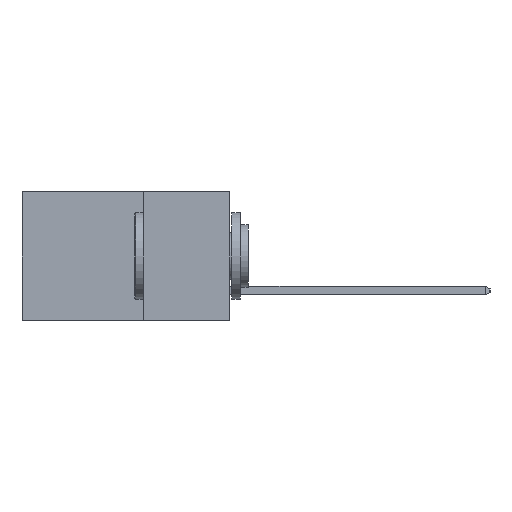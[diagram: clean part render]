
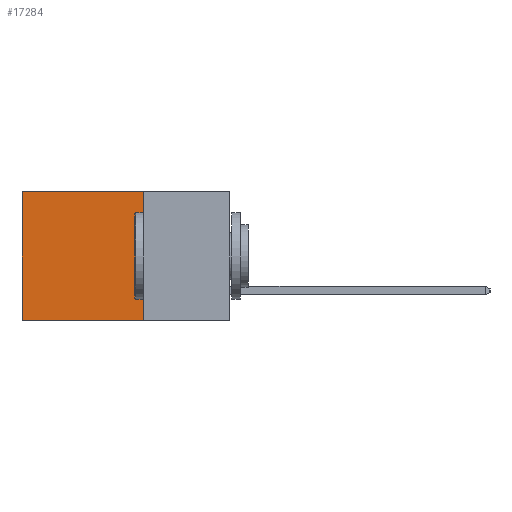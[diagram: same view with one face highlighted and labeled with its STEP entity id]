
A CAD part, left-side view. The second image highlights one B-rep face of the part: STEP entity #17284.
In plain terms, the highlighted planar face has unit normal (-1, 0, 0).
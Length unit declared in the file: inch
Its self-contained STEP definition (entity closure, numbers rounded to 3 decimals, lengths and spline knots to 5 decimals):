
#304 = VERTEX_POINT ( 'NONE', #15848 ) ;
#619 = EDGE_CURVE ( 'NONE', #304, #3793, #16123, .T. ) ;
#997 = FACE_OUTER_BOUND ( 'NONE', #23389, .T. ) ;
#1008 = CARTESIAN_POINT ( 'NONE',  ( 0.2615, 0.6, -0.37 ) ) ;
#1501 = EDGE_CURVE ( 'NONE', #9234, #13480, #11164, .T. ) ;
#1624 = ORIENTED_EDGE ( 'NONE', *, *, #1501, .T. ) ;
#1763 = ORIENTED_EDGE ( 'NONE', *, *, #7703, .T. ) ;
#3793 = VERTEX_POINT ( 'NONE', #11494 ) ;
#4289 = LINE ( 'NONE', #14036, #9132 ) ;
#4417 = VECTOR ( 'NONE', #11997, 39.37008 ) ;
#7703 = EDGE_CURVE ( 'NONE', #304, #9234, #4289, .T. ) ;
#8864 = LINE ( 'NONE', #21607, #14422 ) ;
#9132 = VECTOR ( 'NONE', #13951, 39.37008 ) ;
#9234 = VERTEX_POINT ( 'NONE', #10578 ) ;
#9853 = VECTOR ( 'NONE', #17788, 39.37008 ) ;
#10578 = CARTESIAN_POINT ( 'NONE',  ( 0.2615, 0.6, 0. ) ) ;
#11164 = LINE ( 'NONE', #18100, #9853 ) ;
#11423 = DIRECTION ( 'NONE',  ( 0., 1., 0. ) ) ;
#11494 = CARTESIAN_POINT ( 'NONE',  ( 0.2615, 0.25, -0.37 ) ) ;
#11997 = DIRECTION ( 'NONE',  ( 0., 0., -1. ) ) ;
#12255 = ORIENTED_EDGE ( 'NONE', *, *, #619, .F. ) ;
#12452 = DIRECTION ( 'NONE',  ( 1., 0., 0. ) ) ;
#13480 = VERTEX_POINT ( 'NONE', #1008 ) ;
#13951 = DIRECTION ( 'NONE',  ( 0., 1., 0. ) ) ;
#14036 = CARTESIAN_POINT ( 'NONE',  ( 0.2615, 0.25, 0. ) ) ;
#14422 = VECTOR ( 'NONE', #11423, 39.37008 ) ;
#15316 = ORIENTED_EDGE ( 'NONE', *, *, #17641, .F. ) ;
#15848 = CARTESIAN_POINT ( 'NONE',  ( 0.2615, 0.25, 0. ) ) ;
#16123 = LINE ( 'NONE', #22411, #4417 ) ;
#17284 = ADVANCED_FACE ( 'NONE', ( #997 ), #20579, .F. ) ;
#17641 = EDGE_CURVE ( 'NONE', #3793, #13480, #8864, .T. ) ;
#17788 = DIRECTION ( 'NONE',  ( 0., 0., -1. ) ) ;
#18100 = CARTESIAN_POINT ( 'NONE',  ( 0.2615, 0.6, -0.37 ) ) ;
#18897 = AXIS2_PLACEMENT_3D ( 'NONE', #24582, #12452, #26609 ) ;
#20579 = PLANE ( 'NONE',  #18897 ) ;
#21607 = CARTESIAN_POINT ( 'NONE',  ( 0.2615, 0.25, -0.37 ) ) ;
#22411 = CARTESIAN_POINT ( 'NONE',  ( 0.2615, 0.25, -0.37 ) ) ;
#23389 = EDGE_LOOP ( 'NONE', ( #1624, #15316, #12255, #1763 ) ) ;
#24582 = CARTESIAN_POINT ( 'NONE',  ( 0.2615, 0.25, -0.37 ) ) ;
#26609 = DIRECTION ( 'NONE',  ( 0., 0., -1. ) ) ;
